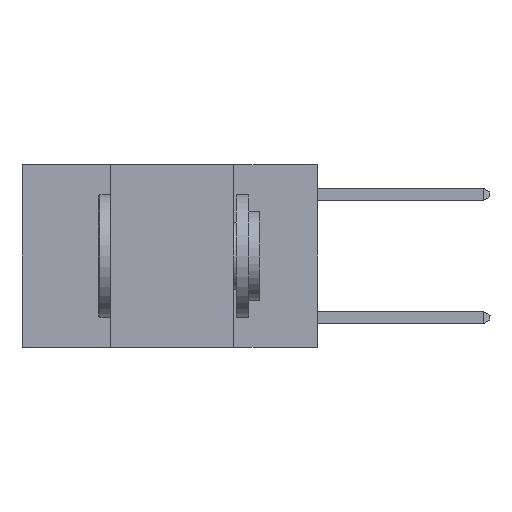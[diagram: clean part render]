
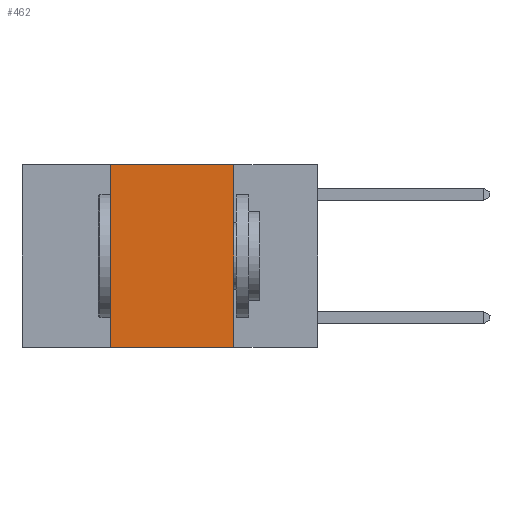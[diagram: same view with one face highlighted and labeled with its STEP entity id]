
A CAD part, left-side view. The second image highlights one B-rep face of the part: STEP entity #462.
In plain terms, the highlighted planar face has unit normal (-1, 0, 0).
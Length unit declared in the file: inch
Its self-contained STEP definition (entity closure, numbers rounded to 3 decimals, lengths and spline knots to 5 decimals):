
#64 = ORIENTED_EDGE ( 'NONE', *, *, #9030, .F. ) ;
#462 = ADVANCED_FACE ( 'NONE', ( #502 ), #9701, .F. ) ;
#502 = FACE_OUTER_BOUND ( 'NONE', #4094, .T. ) ;
#979 = VERTEX_POINT ( 'NONE', #2901 ) ;
#1452 = VERTEX_POINT ( 'NONE', #9755 ) ;
#1685 = CARTESIAN_POINT ( 'NONE',  ( 0., 0.6, 0. ) ) ;
#1750 = VERTEX_POINT ( 'NONE', #2797 ) ;
#2517 = VECTOR ( 'NONE', #3918, 39.37008 ) ;
#2589 = CARTESIAN_POINT ( 'NONE',  ( 0., 0.17, 0. ) ) ;
#2770 = LINE ( 'NONE', #9326, #2517 ) ;
#2797 = CARTESIAN_POINT ( 'NONE',  ( 0., 0.17, -0.37 ) ) ;
#2901 = CARTESIAN_POINT ( 'NONE',  ( 0., 0.42, -0.37 ) ) ;
#3111 = DIRECTION ( 'NONE',  ( 0., 0., 1. ) ) ;
#3165 = LINE ( 'NONE', #3740, #9134 ) ;
#3740 = CARTESIAN_POINT ( 'NONE',  ( 0., 0.6, -0.37 ) ) ;
#3766 = CARTESIAN_POINT ( 'NONE',  ( 0., 0.6, 0. ) ) ;
#3918 = DIRECTION ( 'NONE',  ( 0., 0., -1. ) ) ;
#3925 = VECTOR ( 'NONE', #7655, 39.37008 ) ;
#4094 = EDGE_LOOP ( 'NONE', ( #64, #9004, #5139, #9486 ) ) ;
#4169 = LINE ( 'NONE', #3766, #3925 ) ;
#4238 = DIRECTION ( 'NONE',  ( 0., 0., -1. ) ) ;
#4570 = DIRECTION ( 'NONE',  ( 0., -1., 0. ) ) ;
#4583 = DIRECTION ( 'NONE',  ( 1., 0., 0. ) ) ;
#4767 = CARTESIAN_POINT ( 'NONE',  ( 0., 0.42, 0. ) ) ;
#5139 = ORIENTED_EDGE ( 'NONE', *, *, #8373, .F. ) ;
#5282 = LINE ( 'NONE', #4767, #6614 ) ;
#5689 = VERTEX_POINT ( 'NONE', #2589 ) ;
#6614 = VECTOR ( 'NONE', #3111, 39.37008 ) ;
#7601 = EDGE_CURVE ( 'NONE', #979, #1750, #3165, .T. ) ;
#7655 = DIRECTION ( 'NONE',  ( 0., -1., 0. ) ) ;
#8285 = EDGE_CURVE ( 'NONE', #1452, #5689, #4169, .T. ) ;
#8373 = EDGE_CURVE ( 'NONE', #979, #1452, #5282, .T. ) ;
#9004 = ORIENTED_EDGE ( 'NONE', *, *, #8285, .F. ) ;
#9030 = EDGE_CURVE ( 'NONE', #5689, #1750, #2770, .T. ) ;
#9134 = VECTOR ( 'NONE', #4570, 39.37008 ) ;
#9326 = CARTESIAN_POINT ( 'NONE',  ( 0., 0.17, 0. ) ) ;
#9447 = AXIS2_PLACEMENT_3D ( 'NONE', #1685, #4583, #4238 ) ;
#9486 = ORIENTED_EDGE ( 'NONE', *, *, #7601, .T. ) ;
#9701 = PLANE ( 'NONE',  #9447 ) ;
#9755 = CARTESIAN_POINT ( 'NONE',  ( 0., 0.42, 0. ) ) ;
